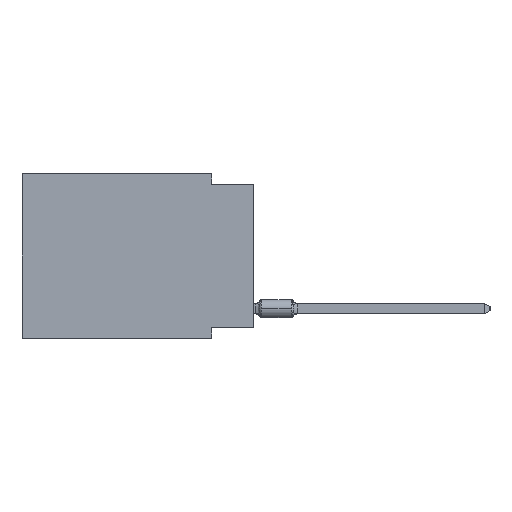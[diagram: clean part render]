
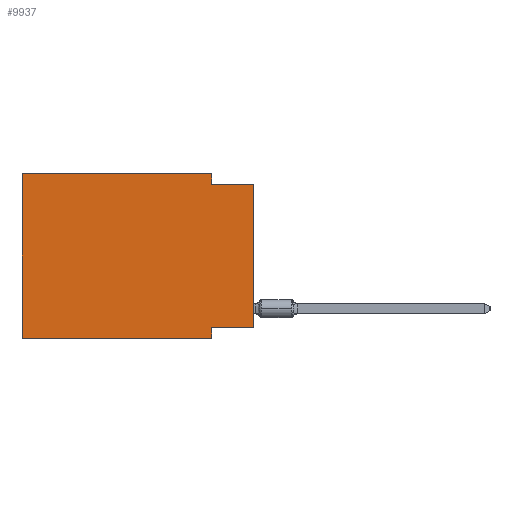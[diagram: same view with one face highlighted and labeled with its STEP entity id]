
A CAD part, left-side view. The second image highlights one B-rep face of the part: STEP entity #9937.
In plain terms, the highlighted planar face has unit normal (-1, 0, 0).
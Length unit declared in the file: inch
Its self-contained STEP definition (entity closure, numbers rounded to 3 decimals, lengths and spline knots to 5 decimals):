
#2413 = EDGE_CURVE ( 'NONE', #24644, #41924, #39711, .T. ) ;
#3249 = CARTESIAN_POINT ( 'NONE',  ( 0., 0., -0.365 ) ) ;
#3269 = VERTEX_POINT ( 'NONE', #37924 ) ;
#4093 = CARTESIAN_POINT ( 'NONE',  ( 0., 0.1, -0.39 ) ) ;
#4199 = ORIENTED_EDGE ( 'NONE', *, *, #2413, .F. ) ;
#4633 = CARTESIAN_POINT ( 'NONE',  ( 0., 0.55, 0. ) ) ;
#5042 = CARTESIAN_POINT ( 'NONE',  ( 0., 0.1, -0.39 ) ) ;
#6025 = VERTEX_POINT ( 'NONE', #17192 ) ;
#6215 = EDGE_CURVE ( 'NONE', #6025, #41924, #7303, .T. ) ;
#7303 = LINE ( 'NONE', #10670, #40497 ) ;
#8307 = LINE ( 'NONE', #18117, #13383 ) ;
#8973 = EDGE_CURVE ( 'NONE', #42977, #3269, #11538, .T. ) ;
#9937 = ADVANCED_FACE ( 'NONE', ( #29239 ), #12671, .F. ) ;
#10177 = VECTOR ( 'NONE', #18096, 39.37008 ) ;
#10670 = CARTESIAN_POINT ( 'NONE',  ( 0., 0., 0. ) ) ;
#11538 = LINE ( 'NONE', #35112, #45374 ) ;
#12047 = DIRECTION ( 'NONE',  ( 0., 1., 0. ) ) ;
#12129 = LINE ( 'NONE', #4093, #36967 ) ;
#12671 = PLANE ( 'NONE',  #45450 ) ;
#12844 = DIRECTION ( 'NONE',  ( 0., 0., -1. ) ) ;
#13379 = CARTESIAN_POINT ( 'NONE',  ( 0., 0., -0.025 ) ) ;
#13383 = VECTOR ( 'NONE', #17879, 39.37008 ) ;
#13628 = ORIENTED_EDGE ( 'NONE', *, *, #15516, .F. ) ;
#13972 = ORIENTED_EDGE ( 'NONE', *, *, #30201, .F. ) ;
#15516 = EDGE_CURVE ( 'NONE', #3269, #43770, #49382, .T. ) ;
#16294 = DIRECTION ( 'NONE',  ( 1., 0., 0. ) ) ;
#16747 = EDGE_LOOP ( 'NONE', ( #35875, #4199, #23471, #13628, #44894, #28839, #13972, #26492 ) ) ;
#17192 = CARTESIAN_POINT ( 'NONE',  ( 0., 0., -0.365 ) ) ;
#17306 = DIRECTION ( 'NONE',  ( 0., 0., -1. ) ) ;
#17469 = EDGE_CURVE ( 'NONE', #43770, #24644, #18175, .T. ) ;
#17819 = EDGE_CURVE ( 'NONE', #42977, #20600, #8307, .T. ) ;
#17879 = DIRECTION ( 'NONE',  ( 0., -1., 0. ) ) ;
#17959 = CARTESIAN_POINT ( 'NONE',  ( 0., 0.1, 0. ) ) ;
#18096 = DIRECTION ( 'NONE',  ( 0., -1., 0. ) ) ;
#18117 = CARTESIAN_POINT ( 'NONE',  ( 0., 0.55, -0.39 ) ) ;
#18175 = LINE ( 'NONE', #38092, #31518 ) ;
#19049 = LINE ( 'NONE', #3249, #40073 ) ;
#20177 = DIRECTION ( 'NONE',  ( 0., 0., -1. ) ) ;
#20600 = VERTEX_POINT ( 'NONE', #5042 ) ;
#23471 = ORIENTED_EDGE ( 'NONE', *, *, #17469, .F. ) ;
#24644 = VERTEX_POINT ( 'NONE', #26789 ) ;
#26089 = VERTEX_POINT ( 'NONE', #48981 ) ;
#26492 = ORIENTED_EDGE ( 'NONE', *, *, #27604, .F. ) ;
#26789 = CARTESIAN_POINT ( 'NONE',  ( 0., 0.1, -0.025 ) ) ;
#27604 = EDGE_CURVE ( 'NONE', #6025, #26089, #19049, .T. ) ;
#28839 = ORIENTED_EDGE ( 'NONE', *, *, #17819, .T. ) ;
#29239 = FACE_OUTER_BOUND ( 'NONE', #16747, .T. ) ;
#29704 = VECTOR ( 'NONE', #36610, 39.37008 ) ;
#30201 = EDGE_CURVE ( 'NONE', #26089, #20600, #12129, .T. ) ;
#31483 = DIRECTION ( 'NONE',  ( 0., 0., 1. ) ) ;
#31518 = VECTOR ( 'NONE', #12844, 39.37008 ) ;
#35112 = CARTESIAN_POINT ( 'NONE',  ( 0., 0.55, 0. ) ) ;
#35875 = ORIENTED_EDGE ( 'NONE', *, *, #6215, .T. ) ;
#36610 = DIRECTION ( 'NONE',  ( 0., -1., 0. ) ) ;
#36967 = VECTOR ( 'NONE', #20177, 39.37008 ) ;
#37526 = CARTESIAN_POINT ( 'NONE',  ( 0., 0.55, 0. ) ) ;
#37924 = CARTESIAN_POINT ( 'NONE',  ( 0., 0.55, 0. ) ) ;
#38092 = CARTESIAN_POINT ( 'NONE',  ( 0., 0.1, 0. ) ) ;
#38871 = DIRECTION ( 'NONE',  ( 0., 0., 1. ) ) ;
#39711 = LINE ( 'NONE', #44343, #29704 ) ;
#40073 = VECTOR ( 'NONE', #12047, 39.37008 ) ;
#40497 = VECTOR ( 'NONE', #38871, 39.37008 ) ;
#41924 = VERTEX_POINT ( 'NONE', #13379 ) ;
#42977 = VERTEX_POINT ( 'NONE', #45229 ) ;
#43770 = VERTEX_POINT ( 'NONE', #17959 ) ;
#44343 = CARTESIAN_POINT ( 'NONE',  ( 0., 0., -0.025 ) ) ;
#44894 = ORIENTED_EDGE ( 'NONE', *, *, #8973, .F. ) ;
#45229 = CARTESIAN_POINT ( 'NONE',  ( 0., 0.55, -0.39 ) ) ;
#45374 = VECTOR ( 'NONE', #31483, 39.37008 ) ;
#45450 = AXIS2_PLACEMENT_3D ( 'NONE', #4633, #16294, #17306 ) ;
#48981 = CARTESIAN_POINT ( 'NONE',  ( 0., 0.1, -0.365 ) ) ;
#49382 = LINE ( 'NONE', #37526, #10177 ) ;
